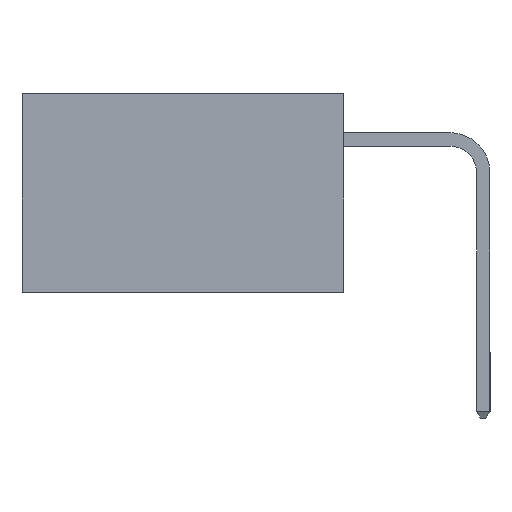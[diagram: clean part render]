
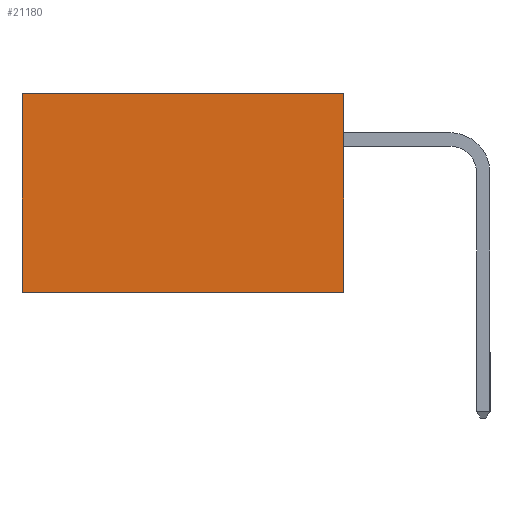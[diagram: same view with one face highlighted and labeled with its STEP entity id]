
A CAD part, left-side view. The second image highlights one B-rep face of the part: STEP entity #21180.
In plain terms, the highlighted planar face has unit normal (-1, 0, 0).
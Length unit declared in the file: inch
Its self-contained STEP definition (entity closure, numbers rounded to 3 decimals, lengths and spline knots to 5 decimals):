
#1377 = CARTESIAN_POINT ( 'NONE',  ( 0.298, 0., 0. ) ) ;
#1905 = ORIENTED_EDGE ( 'NONE', *, *, #10504, .T. ) ;
#3300 = EDGE_CURVE ( 'NONE', #15888, #11373, #14906, .T. ) ;
#3408 = CARTESIAN_POINT ( 'NONE',  ( 0.298, 0., 0. ) ) ;
#4153 = EDGE_LOOP ( 'NONE', ( #10826, #5859, #8433, #1905 ) ) ;
#4361 = DIRECTION ( 'NONE',  ( 0., 0., -1. ) ) ;
#4772 = VECTOR ( 'NONE', #20855, 39.37008 ) ;
#5859 = ORIENTED_EDGE ( 'NONE', *, *, #21028, .F. ) ;
#6708 = CARTESIAN_POINT ( 'NONE',  ( 0.298, 0.6, -0.37 ) ) ;
#6882 = PLANE ( 'NONE',  #20431 ) ;
#7780 = CARTESIAN_POINT ( 'NONE',  ( 0.298, 0.6, 0. ) ) ;
#8043 = VERTEX_POINT ( 'NONE', #6708 ) ;
#8433 = ORIENTED_EDGE ( 'NONE', *, *, #3300, .F. ) ;
#8652 = DIRECTION ( 'NONE',  ( 1., 0., 0. ) ) ;
#9136 = EDGE_CURVE ( 'NONE', #11417, #8043, #10713, .T. ) ;
#10031 = LINE ( 'NONE', #11869, #11432 ) ;
#10504 = EDGE_CURVE ( 'NONE', #15888, #11417, #11479, .T. ) ;
#10713 = LINE ( 'NONE', #7780, #18831 ) ;
#10826 = ORIENTED_EDGE ( 'NONE', *, *, #9136, .T. ) ;
#11373 = VERTEX_POINT ( 'NONE', #19307 ) ;
#11417 = VERTEX_POINT ( 'NONE', #17740 ) ;
#11432 = VECTOR ( 'NONE', #20841, 39.37008 ) ;
#11479 = LINE ( 'NONE', #15807, #4772 ) ;
#11869 = CARTESIAN_POINT ( 'NONE',  ( 0.298, 0., -0.37 ) ) ;
#14906 = LINE ( 'NONE', #3408, #19723 ) ;
#15807 = CARTESIAN_POINT ( 'NONE',  ( 0.298, 0., 0. ) ) ;
#15825 = DIRECTION ( 'NONE',  ( 0., 0., -1. ) ) ;
#15888 = VERTEX_POINT ( 'NONE', #1377 ) ;
#17740 = CARTESIAN_POINT ( 'NONE',  ( 0.298, 0.6, 0. ) ) ;
#18831 = VECTOR ( 'NONE', #4361, 39.37008 ) ;
#19307 = CARTESIAN_POINT ( 'NONE',  ( 0.298, 0., -0.37 ) ) ;
#19468 = CARTESIAN_POINT ( 'NONE',  ( 0.298, 0., 0. ) ) ;
#19723 = VECTOR ( 'NONE', #15825, 39.37008 ) ;
#20431 = AXIS2_PLACEMENT_3D ( 'NONE', #19468, #8652, #21139 ) ;
#20841 = DIRECTION ( 'NONE',  ( 0., 1., 0. ) ) ;
#20855 = DIRECTION ( 'NONE',  ( 0., 1., 0. ) ) ;
#21028 = EDGE_CURVE ( 'NONE', #11373, #8043, #10031, .T. ) ;
#21139 = DIRECTION ( 'NONE',  ( 0., 0., -1. ) ) ;
#21180 = ADVANCED_FACE ( 'NONE', ( #21750 ), #6882, .F. ) ;
#21750 = FACE_OUTER_BOUND ( 'NONE', #4153, .T. ) ;
